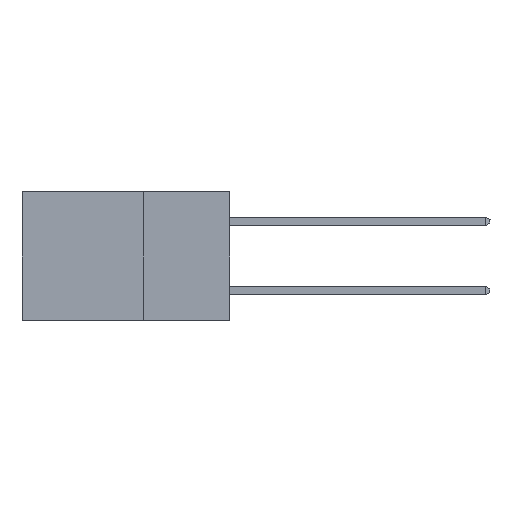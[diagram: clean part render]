
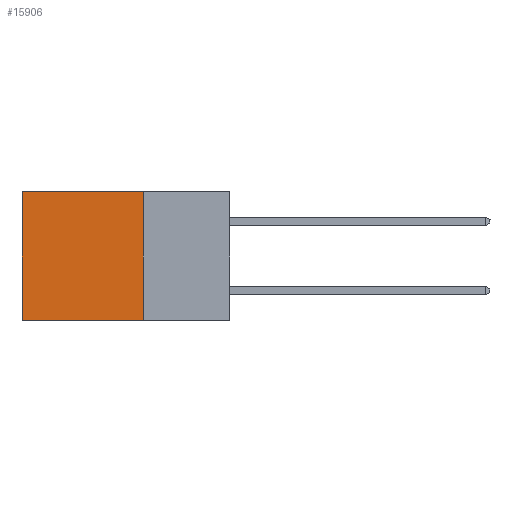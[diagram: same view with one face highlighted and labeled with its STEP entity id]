
A CAD part, left-side view. The second image highlights one B-rep face of the part: STEP entity #15906.
In plain terms, the highlighted planar face has unit normal (-1, 0, 0).
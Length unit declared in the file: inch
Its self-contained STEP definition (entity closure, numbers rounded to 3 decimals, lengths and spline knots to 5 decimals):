
#289 = EDGE_CURVE ( 'NONE', #23562, #2871, #18991, .T. ) ;
#1307 = DIRECTION ( 'NONE',  ( 0., 0., -1. ) ) ;
#1497 = CARTESIAN_POINT ( 'NONE',  ( 0.2615, 0.6, -0.37 ) ) ;
#1688 = VECTOR ( 'NONE', #19734, 39.37008 ) ;
#2871 = VERTEX_POINT ( 'NONE', #24205 ) ;
#3839 = EDGE_CURVE ( 'NONE', #2871, #17293, #12390, .T. ) ;
#4334 = LINE ( 'NONE', #12213, #13343 ) ;
#4819 = CARTESIAN_POINT ( 'NONE',  ( 0.2615, 0.25, -0.37 ) ) ;
#7548 = DIRECTION ( 'NONE',  ( 0., 0., -1. ) ) ;
#7923 = FACE_OUTER_BOUND ( 'NONE', #9939, .T. ) ;
#9716 = VECTOR ( 'NONE', #1307, 39.37008 ) ;
#9939 = EDGE_LOOP ( 'NONE', ( #16288, #18738, #20433, #22515 ) ) ;
#10423 = VECTOR ( 'NONE', #20746, 39.37008 ) ;
#11890 = CARTESIAN_POINT ( 'NONE',  ( 0.2615, 0.25, -0.37 ) ) ;
#12213 = CARTESIAN_POINT ( 'NONE',  ( 0.2615, 0.25, 0. ) ) ;
#12390 = LINE ( 'NONE', #11890, #1688 ) ;
#13343 = VECTOR ( 'NONE', #20058, 39.37008 ) ;
#13723 = DIRECTION ( 'NONE',  ( 1., 0., 0. ) ) ;
#14222 = EDGE_CURVE ( 'NONE', #24544, #17293, #16996, .T. ) ;
#15677 = EDGE_CURVE ( 'NONE', #23562, #24544, #4334, .T. ) ;
#15906 = ADVANCED_FACE ( 'NONE', ( #7923 ), #17723, .F. ) ;
#16288 = ORIENTED_EDGE ( 'NONE', *, *, #14222, .T. ) ;
#16996 = LINE ( 'NONE', #1497, #10423 ) ;
#17293 = VERTEX_POINT ( 'NONE', #19051 ) ;
#17723 = PLANE ( 'NONE',  #20761 ) ;
#18738 = ORIENTED_EDGE ( 'NONE', *, *, #3839, .F. ) ;
#18991 = LINE ( 'NONE', #4819, #9716 ) ;
#19051 = CARTESIAN_POINT ( 'NONE',  ( 0.2615, 0.6, -0.37 ) ) ;
#19734 = DIRECTION ( 'NONE',  ( 0., 1., 0. ) ) ;
#20058 = DIRECTION ( 'NONE',  ( 0., 1., 0. ) ) ;
#20433 = ORIENTED_EDGE ( 'NONE', *, *, #289, .F. ) ;
#20537 = CARTESIAN_POINT ( 'NONE',  ( 0.2615, 0.6, 0. ) ) ;
#20746 = DIRECTION ( 'NONE',  ( 0., 0., -1. ) ) ;
#20761 = AXIS2_PLACEMENT_3D ( 'NONE', #25220, #13723, #7548 ) ;
#20996 = CARTESIAN_POINT ( 'NONE',  ( 0.2615, 0.25, 0. ) ) ;
#22515 = ORIENTED_EDGE ( 'NONE', *, *, #15677, .T. ) ;
#23562 = VERTEX_POINT ( 'NONE', #20996 ) ;
#24205 = CARTESIAN_POINT ( 'NONE',  ( 0.2615, 0.25, -0.37 ) ) ;
#24544 = VERTEX_POINT ( 'NONE', #20537 ) ;
#25220 = CARTESIAN_POINT ( 'NONE',  ( 0.2615, 0.25, -0.37 ) ) ;
